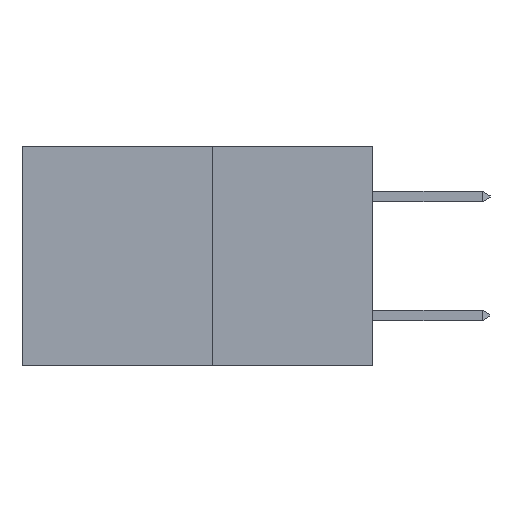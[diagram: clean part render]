
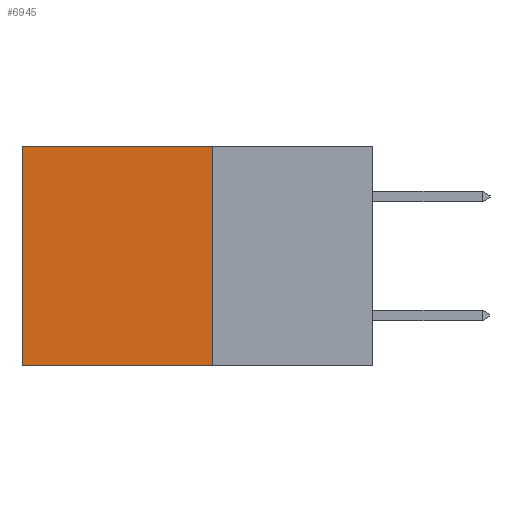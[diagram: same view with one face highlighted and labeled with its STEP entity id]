
A CAD part, left-side view. The second image highlights one B-rep face of the part: STEP entity #6945.
In plain terms, the highlighted planar face has unit normal (-1, 0, 0).
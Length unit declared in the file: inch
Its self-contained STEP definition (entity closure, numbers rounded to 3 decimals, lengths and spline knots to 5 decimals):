
#249 = VECTOR ( 'NONE', #12378, 39.37008 ) ;
#409 = ORIENTED_EDGE ( 'NONE', *, *, #14421, .F. ) ;
#650 = ORIENTED_EDGE ( 'NONE', *, *, #1736, .T. ) ;
#1446 = EDGE_CURVE ( 'NONE', #16672, #17522, #14764, .T. ) ;
#1736 = EDGE_CURVE ( 'NONE', #4590, #16672, #17441, .T. ) ;
#1850 = VECTOR ( 'NONE', #3544, 39.37008 ) ;
#2566 = VECTOR ( 'NONE', #4125, 39.37008 ) ;
#2974 = EDGE_LOOP ( 'NONE', ( #5448, #17964, #409, #650 ) ) ;
#3544 = DIRECTION ( 'NONE',  ( 0., 1., 0. ) ) ;
#4125 = DIRECTION ( 'NONE',  ( 0., 0., -1. ) ) ;
#4226 = LINE ( 'NONE', #9354, #249 ) ;
#4590 = VERTEX_POINT ( 'NONE', #8049 ) ;
#5153 = DIRECTION ( 'NONE',  ( 1., 0., 0. ) ) ;
#5448 = ORIENTED_EDGE ( 'NONE', *, *, #1446, .T. ) ;
#6945 = ADVANCED_FACE ( 'NONE', ( #11359 ), #16754, .F. ) ;
#8049 = CARTESIAN_POINT ( 'NONE',  ( 0.277, 0.27, 0. ) ) ;
#8107 = CARTESIAN_POINT ( 'NONE',  ( 0.277, 0.27, -0.37 ) ) ;
#8899 = CARTESIAN_POINT ( 'NONE',  ( 0.277, 0.59, -0.37 ) ) ;
#8991 = AXIS2_PLACEMENT_3D ( 'NONE', #13955, #5153, #15359 ) ;
#9354 = CARTESIAN_POINT ( 'NONE',  ( 0.277, 0.27, -0.37 ) ) ;
#9502 = CARTESIAN_POINT ( 'NONE',  ( 0.277, 0.27, 0. ) ) ;
#9706 = LINE ( 'NONE', #8107, #17036 ) ;
#10421 = VERTEX_POINT ( 'NONE', #17475 ) ;
#11048 = DIRECTION ( 'NONE',  ( 0., 0., -1. ) ) ;
#11359 = FACE_OUTER_BOUND ( 'NONE', #2974, .T. ) ;
#11905 = CARTESIAN_POINT ( 'NONE',  ( 0.277, 0.59, 0. ) ) ;
#12378 = DIRECTION ( 'NONE',  ( 0., 1., 0. ) ) ;
#13955 = CARTESIAN_POINT ( 'NONE',  ( 0.277, 0.27, -0.37 ) ) ;
#14317 = EDGE_CURVE ( 'NONE', #10421, #17522, #4226, .T. ) ;
#14421 = EDGE_CURVE ( 'NONE', #4590, #10421, #9706, .T. ) ;
#14764 = LINE ( 'NONE', #8899, #2566 ) ;
#15359 = DIRECTION ( 'NONE',  ( 0., 0., -1. ) ) ;
#16672 = VERTEX_POINT ( 'NONE', #11905 ) ;
#16754 = PLANE ( 'NONE',  #8991 ) ;
#17036 = VECTOR ( 'NONE', #11048, 39.37008 ) ;
#17410 = CARTESIAN_POINT ( 'NONE',  ( 0.277, 0.59, -0.37 ) ) ;
#17441 = LINE ( 'NONE', #9502, #1850 ) ;
#17475 = CARTESIAN_POINT ( 'NONE',  ( 0.277, 0.27, -0.37 ) ) ;
#17522 = VERTEX_POINT ( 'NONE', #17410 ) ;
#17964 = ORIENTED_EDGE ( 'NONE', *, *, #14317, .F. ) ;
